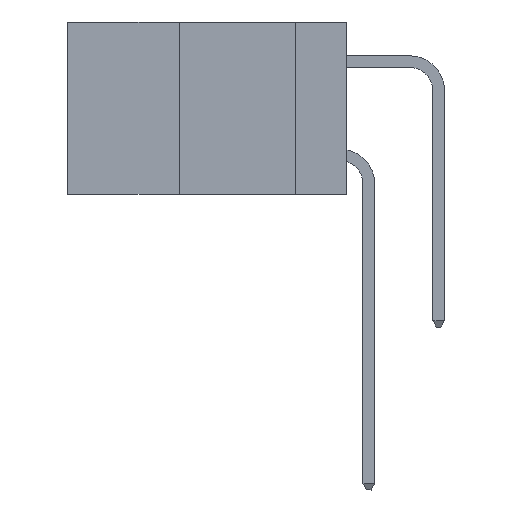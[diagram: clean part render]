
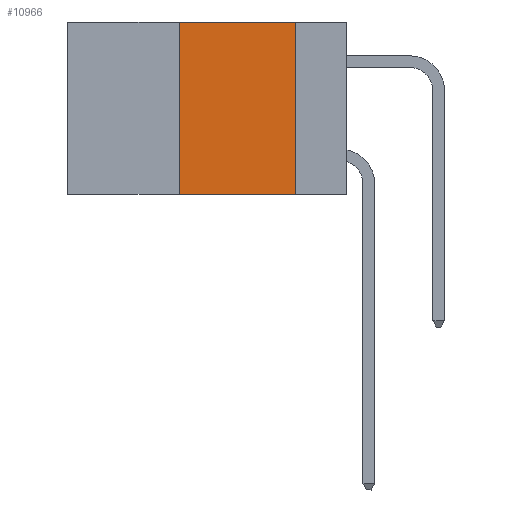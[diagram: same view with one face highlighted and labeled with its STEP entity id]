
A CAD part, left-side view. The second image highlights one B-rep face of the part: STEP entity #10966.
In plain terms, the highlighted planar face has unit normal (-1, 0, 0).
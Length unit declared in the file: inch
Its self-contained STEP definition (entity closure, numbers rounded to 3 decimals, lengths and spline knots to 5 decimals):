
#16 = ORIENTED_EDGE ( 'NONE', *, *, #22269, .F. ) ;
#414 = ORIENTED_EDGE ( 'NONE', *, *, #2642, .F. ) ;
#863 = CARTESIAN_POINT ( 'NONE',  ( 0., 0.36, 0. ) ) ;
#1018 = EDGE_CURVE ( 'NONE', #7186, #10350, #20981, .T. ) ;
#1585 = CARTESIAN_POINT ( 'NONE',  ( 0., 0.6, 0. ) ) ;
#2642 = EDGE_CURVE ( 'NONE', #18530, #21115, #10186, .T. ) ;
#2886 = CARTESIAN_POINT ( 'NONE',  ( 0., 0.11, 0. ) ) ;
#2985 = CARTESIAN_POINT ( 'NONE',  ( 0., 0.6, -0.37 ) ) ;
#4645 = DIRECTION ( 'NONE',  ( 0., 0., -1. ) ) ;
#5168 = CARTESIAN_POINT ( 'NONE',  ( 0., 0.36, 0. ) ) ;
#6302 = DIRECTION ( 'NONE',  ( 0., -1., 0. ) ) ;
#6437 = ORIENTED_EDGE ( 'NONE', *, *, #18910, .T. ) ;
#7186 = VERTEX_POINT ( 'NONE', #19950 ) ;
#9815 = ORIENTED_EDGE ( 'NONE', *, *, #1018, .F. ) ;
#9937 = LINE ( 'NONE', #2985, #22633 ) ;
#10057 = DIRECTION ( 'NONE',  ( 0., -1., 0. ) ) ;
#10186 = LINE ( 'NONE', #2886, #22271 ) ;
#10350 = VERTEX_POINT ( 'NONE', #863 ) ;
#10966 = ADVANCED_FACE ( 'NONE', ( #20459 ), #20676, .F. ) ;
#12993 = VECTOR ( 'NONE', #6302, 39.37008 ) ;
#14131 = VECTOR ( 'NONE', #15892, 39.37008 ) ;
#15892 = DIRECTION ( 'NONE',  ( 0., 0., 1. ) ) ;
#16331 = CARTESIAN_POINT ( 'NONE',  ( 0., 0.11, 0. ) ) ;
#16935 = LINE ( 'NONE', #20521, #12993 ) ;
#17203 = EDGE_LOOP ( 'NONE', ( #414, #16, #9815, #6437 ) ) ;
#17214 = DIRECTION ( 'NONE',  ( 0., 0., -1. ) ) ;
#17713 = CARTESIAN_POINT ( 'NONE',  ( 0., 0.11, -0.37 ) ) ;
#18530 = VERTEX_POINT ( 'NONE', #16331 ) ;
#18910 = EDGE_CURVE ( 'NONE', #7186, #21115, #9937, .T. ) ;
#19049 = DIRECTION ( 'NONE',  ( 1., 0., 0. ) ) ;
#19950 = CARTESIAN_POINT ( 'NONE',  ( 0., 0.36, -0.37 ) ) ;
#20459 = FACE_OUTER_BOUND ( 'NONE', #17203, .T. ) ;
#20521 = CARTESIAN_POINT ( 'NONE',  ( 0., 0.6, 0. ) ) ;
#20676 = PLANE ( 'NONE',  #22061 ) ;
#20981 = LINE ( 'NONE', #5168, #14131 ) ;
#21115 = VERTEX_POINT ( 'NONE', #17713 ) ;
#22061 = AXIS2_PLACEMENT_3D ( 'NONE', #1585, #19049, #17214 ) ;
#22269 = EDGE_CURVE ( 'NONE', #10350, #18530, #16935, .T. ) ;
#22271 = VECTOR ( 'NONE', #4645, 39.37008 ) ;
#22633 = VECTOR ( 'NONE', #10057, 39.37008 ) ;
